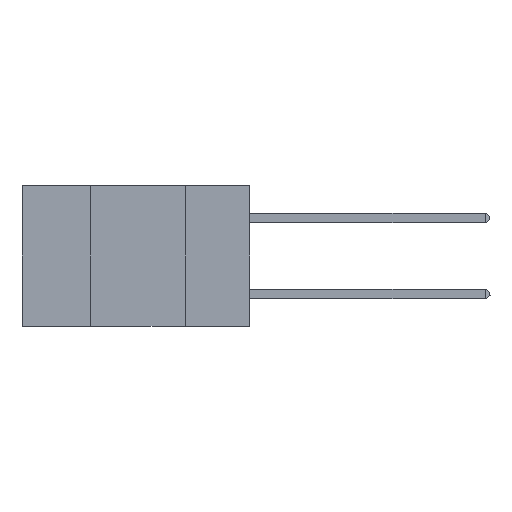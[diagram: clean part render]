
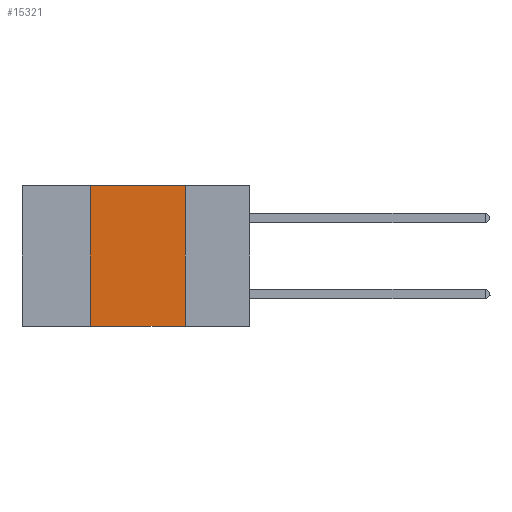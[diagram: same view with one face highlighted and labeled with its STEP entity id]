
A CAD part, left-side view. The second image highlights one B-rep face of the part: STEP entity #15321.
In plain terms, the highlighted planar face has unit normal (-1, 0, 0).
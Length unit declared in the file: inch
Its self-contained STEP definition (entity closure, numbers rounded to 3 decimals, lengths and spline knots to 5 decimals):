
#606 = DIRECTION ( 'NONE',  ( 0., -1., 0. ) ) ;
#821 = DIRECTION ( 'NONE',  ( 0., 0., -1. ) ) ;
#1208 = VECTOR ( 'NONE', #4343, 39.37008 ) ;
#1803 = VECTOR ( 'NONE', #5029, 39.37008 ) ;
#1936 = CARTESIAN_POINT ( 'NONE',  ( 0., 0.6, -0.37 ) ) ;
#3441 = VERTEX_POINT ( 'NONE', #5149 ) ;
#4343 = DIRECTION ( 'NONE',  ( 0., 0., -1. ) ) ;
#4611 = VERTEX_POINT ( 'NONE', #6614 ) ;
#5029 = DIRECTION ( 'NONE',  ( 0., 0., 1. ) ) ;
#5138 = CARTESIAN_POINT ( 'NONE',  ( 0., 0.42, 0. ) ) ;
#5149 = CARTESIAN_POINT ( 'NONE',  ( 0., 0.17, -0.37 ) ) ;
#5212 = DIRECTION ( 'NONE',  ( 1., 0., 0. ) ) ;
#5564 = ORIENTED_EDGE ( 'NONE', *, *, #8542, .F. ) ;
#6614 = CARTESIAN_POINT ( 'NONE',  ( 0., 0.17, 0. ) ) ;
#8425 = DIRECTION ( 'NONE',  ( 0., -1., 0. ) ) ;
#8542 = EDGE_CURVE ( 'NONE', #4611, #3441, #10123, .T. ) ;
#8973 = CARTESIAN_POINT ( 'NONE',  ( 0., 0.42, 0. ) ) ;
#9147 = CARTESIAN_POINT ( 'NONE',  ( 0., 0.42, -0.37 ) ) ;
#9545 = EDGE_CURVE ( 'NONE', #10294, #4611, #15223, .T. ) ;
#9725 = CARTESIAN_POINT ( 'NONE',  ( 0., 0.17, 0. ) ) ;
#9768 = FACE_OUTER_BOUND ( 'NONE', #10691, .T. ) ;
#9901 = ORIENTED_EDGE ( 'NONE', *, *, #14713, .T. ) ;
#10002 = VECTOR ( 'NONE', #606, 39.37008 ) ;
#10123 = LINE ( 'NONE', #9725, #1208 ) ;
#10193 = ORIENTED_EDGE ( 'NONE', *, *, #9545, .F. ) ;
#10294 = VERTEX_POINT ( 'NONE', #8973 ) ;
#10691 = EDGE_LOOP ( 'NONE', ( #5564, #10193, #12735, #9901 ) ) ;
#11416 = VERTEX_POINT ( 'NONE', #9147 ) ;
#12735 = ORIENTED_EDGE ( 'NONE', *, *, #13412, .F. ) ;
#13098 = AXIS2_PLACEMENT_3D ( 'NONE', #14780, #5212, #821 ) ;
#13349 = PLANE ( 'NONE',  #13098 ) ;
#13412 = EDGE_CURVE ( 'NONE', #11416, #10294, #17246, .T. ) ;
#13426 = LINE ( 'NONE', #1936, #10002 ) ;
#13449 = CARTESIAN_POINT ( 'NONE',  ( 0., 0.6, 0. ) ) ;
#14343 = VECTOR ( 'NONE', #8425, 39.37008 ) ;
#14713 = EDGE_CURVE ( 'NONE', #11416, #3441, #13426, .T. ) ;
#14780 = CARTESIAN_POINT ( 'NONE',  ( 0., 0.6, 0. ) ) ;
#15223 = LINE ( 'NONE', #13449, #14343 ) ;
#15321 = ADVANCED_FACE ( 'NONE', ( #9768 ), #13349, .F. ) ;
#17246 = LINE ( 'NONE', #5138, #1803 ) ;
